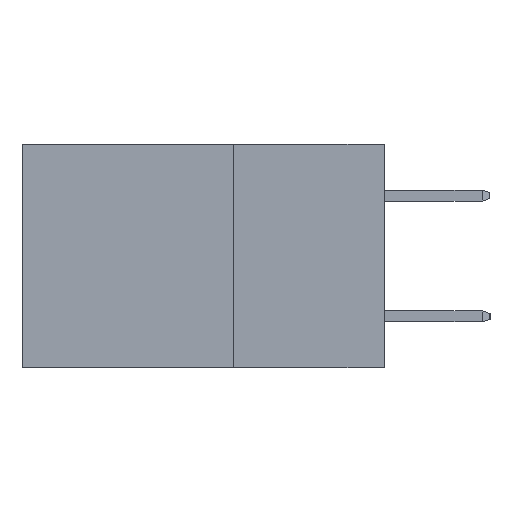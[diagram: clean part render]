
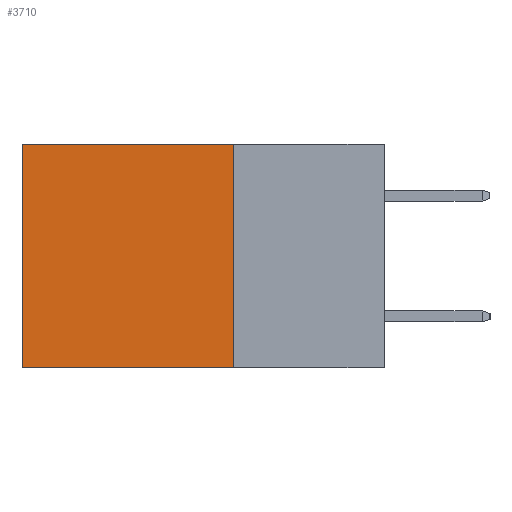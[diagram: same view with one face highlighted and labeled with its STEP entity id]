
A CAD part, left-side view. The second image highlights one B-rep face of the part: STEP entity #3710.
In plain terms, the highlighted planar face has unit normal (-1, 0, 0).
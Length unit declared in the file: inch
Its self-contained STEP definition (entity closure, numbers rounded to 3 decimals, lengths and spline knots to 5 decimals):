
#13 = ORIENTED_EDGE ( 'NONE', *, *, #3365, .T. ) ;
#181 = EDGE_CURVE ( 'NONE', #1261, #1842, #1977, .T. ) ;
#463 = CARTESIAN_POINT ( 'NONE',  ( 0.2615, 0.25, 0. ) ) ;
#1032 = CARTESIAN_POINT ( 'NONE',  ( 0.2615, 0.25, -0.37 ) ) ;
#1099 = LINE ( 'NONE', #463, #10087 ) ;
#1236 = ORIENTED_EDGE ( 'NONE', *, *, #181, .F. ) ;
#1261 = VERTEX_POINT ( 'NONE', #3672 ) ;
#1411 = VERTEX_POINT ( 'NONE', #6705 ) ;
#1610 = ORIENTED_EDGE ( 'NONE', *, *, #10412, .T. ) ;
#1842 = VERTEX_POINT ( 'NONE', #1032 ) ;
#1977 = LINE ( 'NONE', #7071, #3713 ) ;
#2004 = ORIENTED_EDGE ( 'NONE', *, *, #5933, .F. ) ;
#2152 = CARTESIAN_POINT ( 'NONE',  ( 0.2615, 0.6, -0.37 ) ) ;
#2199 = DIRECTION ( 'NONE',  ( 0., 0., -1. ) ) ;
#2573 = LINE ( 'NONE', #4858, #6800 ) ;
#3365 = EDGE_CURVE ( 'NONE', #4604, #1411, #4299, .T. ) ;
#3672 = CARTESIAN_POINT ( 'NONE',  ( 0.2615, 0.25, 0. ) ) ;
#3710 = ADVANCED_FACE ( 'NONE', ( #10380 ), #9605, .F. ) ;
#3713 = VECTOR ( 'NONE', #7031, 39.37008 ) ;
#4299 = LINE ( 'NONE', #2152, #6269 ) ;
#4604 = VERTEX_POINT ( 'NONE', #5263 ) ;
#4858 = CARTESIAN_POINT ( 'NONE',  ( 0.2615, 0.25, -0.37 ) ) ;
#5263 = CARTESIAN_POINT ( 'NONE',  ( 0.2615, 0.6, 0. ) ) ;
#5404 = DIRECTION ( 'NONE',  ( 0., 1., 0. ) ) ;
#5933 = EDGE_CURVE ( 'NONE', #1842, #1411, #2573, .T. ) ;
#6269 = VECTOR ( 'NONE', #2199, 39.37008 ) ;
#6705 = CARTESIAN_POINT ( 'NONE',  ( 0.2615, 0.6, -0.37 ) ) ;
#6800 = VECTOR ( 'NONE', #8134, 39.37008 ) ;
#7031 = DIRECTION ( 'NONE',  ( 0., 0., -1. ) ) ;
#7071 = CARTESIAN_POINT ( 'NONE',  ( 0.2615, 0.25, -0.37 ) ) ;
#7789 = AXIS2_PLACEMENT_3D ( 'NONE', #9435, #9382, #9379 ) ;
#8134 = DIRECTION ( 'NONE',  ( 0., 1., 0. ) ) ;
#9142 = EDGE_LOOP ( 'NONE', ( #13, #2004, #1236, #1610 ) ) ;
#9379 = DIRECTION ( 'NONE',  ( 0., 0., -1. ) ) ;
#9382 = DIRECTION ( 'NONE',  ( 1., 0., 0. ) ) ;
#9435 = CARTESIAN_POINT ( 'NONE',  ( 0.2615, 0.25, -0.37 ) ) ;
#9605 = PLANE ( 'NONE',  #7789 ) ;
#10087 = VECTOR ( 'NONE', #5404, 39.37008 ) ;
#10380 = FACE_OUTER_BOUND ( 'NONE', #9142, .T. ) ;
#10412 = EDGE_CURVE ( 'NONE', #1261, #4604, #1099, .T. ) ;
